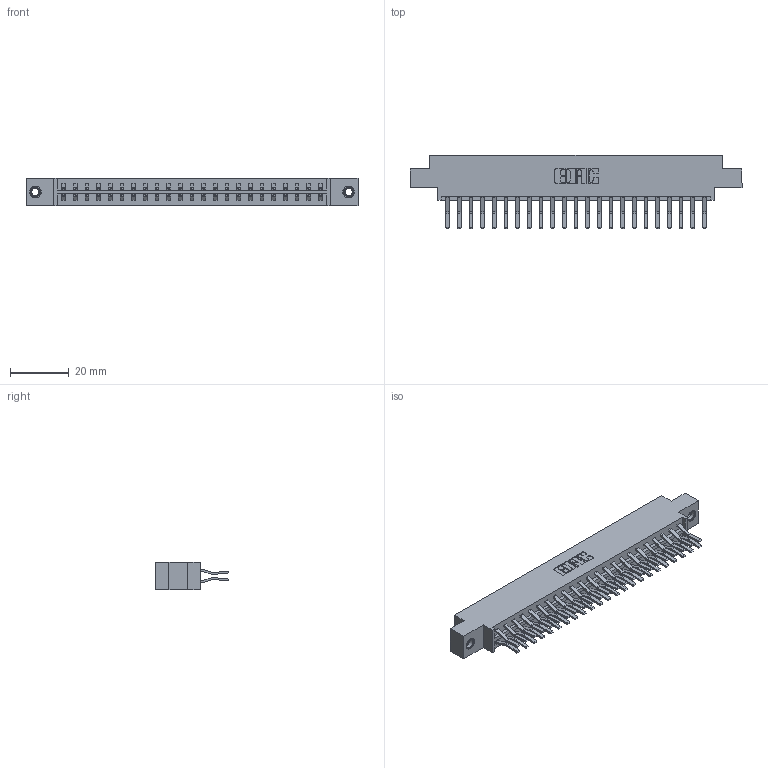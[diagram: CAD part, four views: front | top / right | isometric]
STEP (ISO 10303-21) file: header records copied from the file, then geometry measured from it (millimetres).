
FILE_DESCRIPTION (( 'STEP AP203' ), '1' );
FILE_NAME ('333-046-560-807.STEP', '2018-08-03T23:03:31', ( '' ), ( '' ), 'SwSTEP 2.0', 'SolidWorks 2016', '' );
FILE_SCHEMA (( 'CONFIG_CONTROL_DESIGN' ));
Length unit declared in the file: inch
Products named in the file (4): 333 Part_Offset - .156 Dia - TI; 345-292-001_560 Tail; 345-250-001_345-250-005-103; 333-046-560-807
Assembly tree (49 placements, depth 2):
  333-046-560-807
    333 Part_Offset - .156 Dia - TI
    345-292-001_560 Tail  x46
    345-250-001_345-250-005-103  x2
Bounding box: 112.67 x 24.78 x 9.4 mm (x, y, z)
Volume: 11385.9 mm3; surface area: 14371.9 mm2
Topology: 49 solids, 49 shells, 2662 faces, 7865 edges, 5174 vertices
Faces by surface type: plane 1762, cylinder 884, cone 12, torus 4
Entity records: 18660 total; most frequent: CARTESIAN_POINT 3101, ORIENTED_EDGE 3030, DIRECTION 2717, EDGE_CURVE 1515, LINE 1363, VECTOR 1363, VERTEX_POINT 1004, AXIS2_PLACEMENT_3D 677
